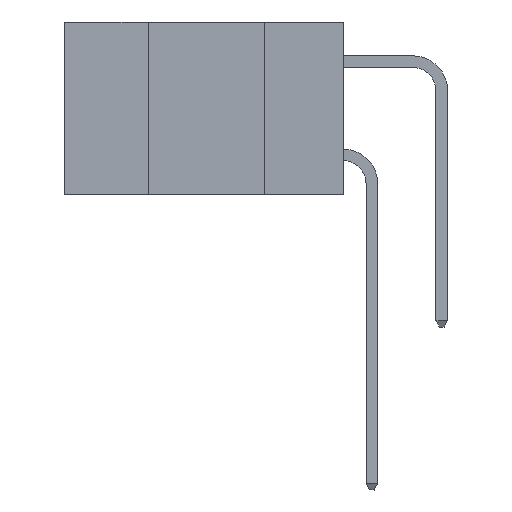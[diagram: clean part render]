
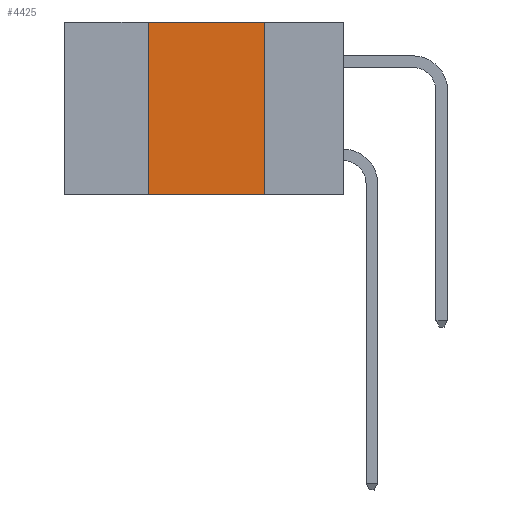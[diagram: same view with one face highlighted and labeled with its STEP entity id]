
A CAD part, left-side view. The second image highlights one B-rep face of the part: STEP entity #4425.
In plain terms, the highlighted planar face has unit normal (-1, 0, 0).
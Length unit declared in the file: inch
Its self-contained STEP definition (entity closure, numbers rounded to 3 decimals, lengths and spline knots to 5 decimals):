
#195 = DIRECTION ( 'NONE',  ( 0., -1., 0. ) ) ;
#273 = PLANE ( 'NONE',  #2495 ) ;
#326 = ORIENTED_EDGE ( 'NONE', *, *, #1948, .F. ) ;
#637 = DIRECTION ( 'NONE',  ( 0., 0., 1. ) ) ;
#1056 = EDGE_CURVE ( 'NONE', #11120, #7343, #11080, .T. ) ;
#1127 = CARTESIAN_POINT ( 'NONE',  ( 0., 0.6, 0. ) ) ;
#1179 = CARTESIAN_POINT ( 'NONE',  ( 0., 0.17, -0.37 ) ) ;
#1187 = FACE_OUTER_BOUND ( 'NONE', #2567, .T. ) ;
#1221 = VECTOR ( 'NONE', #6487, 39.37008 ) ;
#1426 = CARTESIAN_POINT ( 'NONE',  ( 0., 0.42, -0.37 ) ) ;
#1561 = EDGE_CURVE ( 'NONE', #8923, #11477, #8453, .T. ) ;
#1948 = EDGE_CURVE ( 'NONE', #11477, #7343, #9965, .T. ) ;
#2015 = VECTOR ( 'NONE', #195, 39.37008 ) ;
#2495 = AXIS2_PLACEMENT_3D ( 'NONE', #1127, #9315, #4865 ) ;
#2567 = EDGE_LOOP ( 'NONE', ( #326, #11594, #2984, #6348 ) ) ;
#2754 = CARTESIAN_POINT ( 'NONE',  ( 0., 0.6, -0.37 ) ) ;
#2984 = ORIENTED_EDGE ( 'NONE', *, *, #7011, .F. ) ;
#3346 = CARTESIAN_POINT ( 'NONE',  ( 0., 0.17, 0. ) ) ;
#3668 = VECTOR ( 'NONE', #637, 39.37008 ) ;
#4425 = ADVANCED_FACE ( 'NONE', ( #1187 ), #273, .F. ) ;
#4865 = DIRECTION ( 'NONE',  ( 0., 0., -1. ) ) ;
#5261 = CARTESIAN_POINT ( 'NONE',  ( 0., 0.42, -0.37 ) ) ;
#5373 = DIRECTION ( 'NONE',  ( 0., 0., -1. ) ) ;
#6348 = ORIENTED_EDGE ( 'NONE', *, *, #1056, .T. ) ;
#6487 = DIRECTION ( 'NONE',  ( 0., -1., 0. ) ) ;
#6534 = CARTESIAN_POINT ( 'NONE',  ( 0., 0.6, 0. ) ) ;
#7011 = EDGE_CURVE ( 'NONE', #11120, #8923, #11459, .T. ) ;
#7302 = VECTOR ( 'NONE', #5373, 39.37008 ) ;
#7343 = VERTEX_POINT ( 'NONE', #1179 ) ;
#8453 = LINE ( 'NONE', #6534, #2015 ) ;
#8923 = VERTEX_POINT ( 'NONE', #10651 ) ;
#9172 = CARTESIAN_POINT ( 'NONE',  ( 0., 0.17, -0.37 ) ) ;
#9315 = DIRECTION ( 'NONE',  ( 1., 0., 0. ) ) ;
#9965 = LINE ( 'NONE', #9172, #7302 ) ;
#10651 = CARTESIAN_POINT ( 'NONE',  ( 0., 0.42, 0. ) ) ;
#11080 = LINE ( 'NONE', #2754, #1221 ) ;
#11120 = VERTEX_POINT ( 'NONE', #5261 ) ;
#11459 = LINE ( 'NONE', #1426, #3668 ) ;
#11477 = VERTEX_POINT ( 'NONE', #3346 ) ;
#11594 = ORIENTED_EDGE ( 'NONE', *, *, #1561, .F. ) ;
